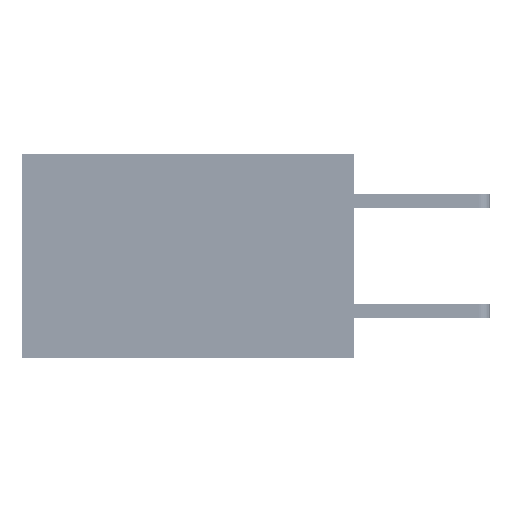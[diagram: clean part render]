
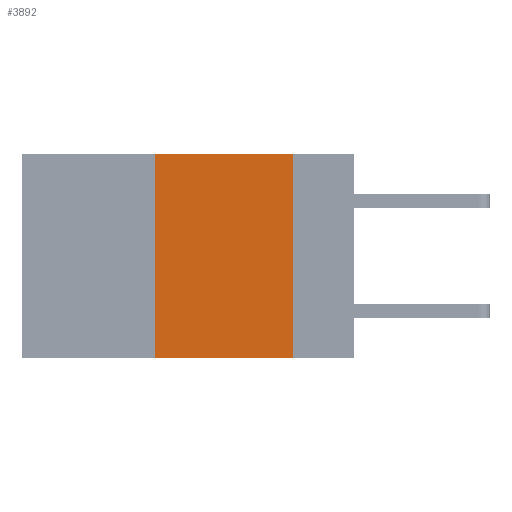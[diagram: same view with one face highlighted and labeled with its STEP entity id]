
A CAD part, left-side view. The second image highlights one B-rep face of the part: STEP entity #3892.
In plain terms, the highlighted planar face has unit normal (-1, 0, 0).
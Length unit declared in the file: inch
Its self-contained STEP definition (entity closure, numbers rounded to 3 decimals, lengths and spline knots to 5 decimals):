
#289 = VECTOR ( 'NONE', #48639, 39.37008 ) ;
#980 = EDGE_CURVE ( 'NONE', #16375, #18471, #5477, .T. ) ;
#1577 = AXIS2_PLACEMENT_3D ( 'NONE', #15985, #28590, #44519 ) ;
#2413 = CARTESIAN_POINT ( 'NONE',  ( 0., 0.11, 0. ) ) ;
#3122 = ORIENTED_EDGE ( 'NONE', *, *, #980, .F. ) ;
#3750 = CARTESIAN_POINT ( 'NONE',  ( 0., 0.6, -0.37 ) ) ;
#3892 = ADVANCED_FACE ( 'NONE', ( #37976 ), #7796, .F. ) ;
#5477 = LINE ( 'NONE', #50725, #40363 ) ;
#7796 = PLANE ( 'NONE',  #1577 ) ;
#9549 = EDGE_CURVE ( 'NONE', #18471, #43161, #22522, .T. ) ;
#10323 = LINE ( 'NONE', #26950, #32431 ) ;
#14687 = ORIENTED_EDGE ( 'NONE', *, *, #9549, .F. ) ;
#15985 = CARTESIAN_POINT ( 'NONE',  ( 0., 0.6, 0. ) ) ;
#16375 = VERTEX_POINT ( 'NONE', #36903 ) ;
#18421 = EDGE_CURVE ( 'NONE', #41751, #43161, #47876, .T. ) ;
#18471 = VERTEX_POINT ( 'NONE', #44893 ) ;
#20730 = CARTESIAN_POINT ( 'NONE',  ( 0., 0.11, -0.37 ) ) ;
#21652 = EDGE_LOOP ( 'NONE', ( #14687, #3122, #36770, #30664 ) ) ;
#22309 = EDGE_CURVE ( 'NONE', #41751, #16375, #10323, .T. ) ;
#22522 = LINE ( 'NONE', #2413, #31410 ) ;
#26460 = DIRECTION ( 'NONE',  ( 0., -1., 0. ) ) ;
#26950 = CARTESIAN_POINT ( 'NONE',  ( 0., 0.36, 0. ) ) ;
#28590 = DIRECTION ( 'NONE',  ( 1., 0., 0. ) ) ;
#30664 = ORIENTED_EDGE ( 'NONE', *, *, #18421, .T. ) ;
#31410 = VECTOR ( 'NONE', #46768, 39.37008 ) ;
#32034 = DIRECTION ( 'NONE',  ( 0., 0., 1. ) ) ;
#32431 = VECTOR ( 'NONE', #32034, 39.37008 ) ;
#36770 = ORIENTED_EDGE ( 'NONE', *, *, #22309, .F. ) ;
#36903 = CARTESIAN_POINT ( 'NONE',  ( 0., 0.36, 0. ) ) ;
#37976 = FACE_OUTER_BOUND ( 'NONE', #21652, .T. ) ;
#40363 = VECTOR ( 'NONE', #26460, 39.37008 ) ;
#41751 = VERTEX_POINT ( 'NONE', #50964 ) ;
#43161 = VERTEX_POINT ( 'NONE', #20730 ) ;
#44519 = DIRECTION ( 'NONE',  ( 0., 0., -1. ) ) ;
#44893 = CARTESIAN_POINT ( 'NONE',  ( 0., 0.11, 0. ) ) ;
#46768 = DIRECTION ( 'NONE',  ( 0., 0., -1. ) ) ;
#47876 = LINE ( 'NONE', #3750, #289 ) ;
#48639 = DIRECTION ( 'NONE',  ( 0., -1., 0. ) ) ;
#50725 = CARTESIAN_POINT ( 'NONE',  ( 0., 0.6, 0. ) ) ;
#50964 = CARTESIAN_POINT ( 'NONE',  ( 0., 0.36, -0.37 ) ) ;
